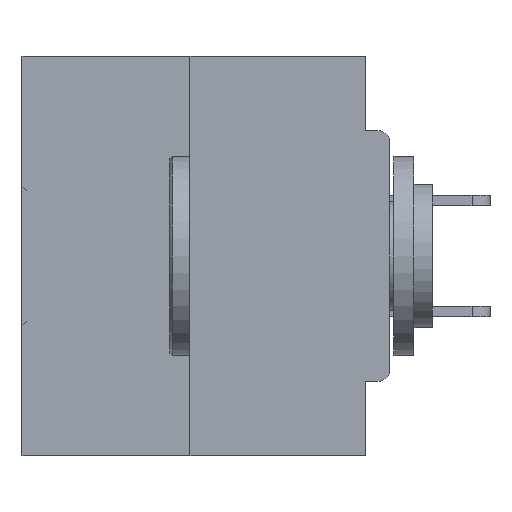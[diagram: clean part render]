
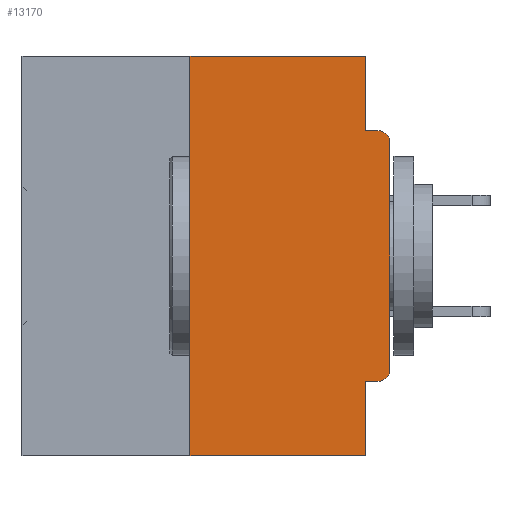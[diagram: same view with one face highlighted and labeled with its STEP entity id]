
A CAD part, left-side view. The second image highlights one B-rep face of the part: STEP entity #13170.
In plain terms, the highlighted planar face has unit normal (-1, 0, 0).
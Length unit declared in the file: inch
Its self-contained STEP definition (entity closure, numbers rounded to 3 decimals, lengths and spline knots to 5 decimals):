
#78 = DIRECTION ( 'NONE',  ( 0., 0., -1. ) ) ;
#475 = EDGE_CURVE ( 'NONE', #14964, #7353, #18288, .T. ) ;
#890 = DIRECTION ( 'NONE',  ( 0., 0., -1. ) ) ;
#1221 = CARTESIAN_POINT ( 'NONE',  ( 0., 0.46, -0.5 ) ) ;
#1668 = EDGE_CURVE ( 'NONE', #23211, #14253, #40710, .T. ) ;
#3344 = EDGE_CURVE ( 'NONE', #44906, #28571, #44698, .T. ) ;
#4486 = AXIS2_PLACEMENT_3D ( 'NONE', #15875, #8685, #5326 ) ;
#4583 = VECTOR ( 'NONE', #78, 39.37008 ) ;
#4726 = LINE ( 'NONE', #22509, #44784 ) ;
#5304 = CARTESIAN_POINT ( 'NONE',  ( 0., 0.25, 0. ) ) ;
#5326 = DIRECTION ( 'NONE',  ( 0., 0., -1. ) ) ;
#5459 = DIRECTION ( 'NONE',  ( 0., 0., 1. ) ) ;
#5738 = CARTESIAN_POINT ( 'NONE',  ( 0., 0.015, -0.1085 ) ) ;
#5760 = LINE ( 'NONE', #10376, #6853 ) ;
#6853 = VECTOR ( 'NONE', #42630, 39.37008 ) ;
#7054 = ORIENTED_EDGE ( 'NONE', *, *, #43190, .F. ) ;
#7353 = VERTEX_POINT ( 'NONE', #10066 ) ;
#8255 = VERTEX_POINT ( 'NONE', #42864 ) ;
#8685 = DIRECTION ( 'NONE',  ( -1., 0., 0. ) ) ;
#8760 = DIRECTION ( 'NONE',  ( 0., -1., 0. ) ) ;
#10066 = CARTESIAN_POINT ( 'NONE',  ( 0., 0.015, -0.0935 ) ) ;
#10376 = CARTESIAN_POINT ( 'NONE',  ( 0., 0.031, 0. ) ) ;
#10467 = VECTOR ( 'NONE', #25319, 39.37008 ) ;
#10963 = ORIENTED_EDGE ( 'NONE', *, *, #11370, .T. ) ;
#11117 = CARTESIAN_POINT ( 'NONE',  ( 0., 0.031, -0.5 ) ) ;
#11202 = DIRECTION ( 'NONE',  ( 0., 1., 0. ) ) ;
#11370 = EDGE_CURVE ( 'NONE', #8255, #14964, #37147, .T. ) ;
#12118 = AXIS2_PLACEMENT_3D ( 'NONE', #5738, #40565, #19067 ) ;
#12357 = EDGE_CURVE ( 'NONE', #30990, #26503, #5760, .T. ) ;
#12519 = LINE ( 'NONE', #40222, #41104 ) ;
#13170 = ADVANCED_FACE ( 'NONE', ( #38039 ), #38951, .F. ) ;
#13207 = ORIENTED_EDGE ( 'NONE', *, *, #20850, .T. ) ;
#14200 = EDGE_CURVE ( 'NONE', #23211, #28475, #35765, .T. ) ;
#14253 = VERTEX_POINT ( 'NONE', #11117 ) ;
#14556 = AXIS2_PLACEMENT_3D ( 'NONE', #17894, #42499, #890 ) ;
#14964 = VERTEX_POINT ( 'NONE', #22464 ) ;
#15875 = CARTESIAN_POINT ( 'NONE',  ( 0., 0.015, -0.3915 ) ) ;
#16377 = CARTESIAN_POINT ( 'NONE',  ( 0., 0.031, 0. ) ) ;
#17894 = CARTESIAN_POINT ( 'NONE',  ( 0., 0.46, 0. ) ) ;
#18135 = ORIENTED_EDGE ( 'NONE', *, *, #3344, .F. ) ;
#18288 = CIRCLE ( 'NONE', #12118, 0.015 ) ;
#19067 = DIRECTION ( 'NONE',  ( 0., 0., -1. ) ) ;
#20060 = CIRCLE ( 'NONE', #4486, 0.015 ) ;
#20195 = ORIENTED_EDGE ( 'NONE', *, *, #475, .T. ) ;
#20850 = EDGE_CURVE ( 'NONE', #44906, #8255, #20060, .T. ) ;
#21730 = ORIENTED_EDGE ( 'NONE', *, *, #38142, .F. ) ;
#22464 = CARTESIAN_POINT ( 'NONE',  ( 0., 0., -0.1085 ) ) ;
#22509 = CARTESIAN_POINT ( 'NONE',  ( 0., 0.46, 0. ) ) ;
#23211 = VERTEX_POINT ( 'NONE', #44111 ) ;
#23949 = CARTESIAN_POINT ( 'NONE',  ( 0., 0.015, -0.4065 ) ) ;
#23973 = VECTOR ( 'NONE', #28690, 39.37008 ) ;
#24333 = LINE ( 'NONE', #42291, #4583 ) ;
#24680 = EDGE_LOOP ( 'NONE', ( #21730, #38659, #35243, #7054, #18135, #13207, #10963, #20195, #37753, #43602 ) ) ;
#25319 = DIRECTION ( 'NONE',  ( 0., -1., 0. ) ) ;
#25388 = EDGE_CURVE ( 'NONE', #26503, #7353, #12519, .T. ) ;
#26503 = VERTEX_POINT ( 'NONE', #33304 ) ;
#28475 = VERTEX_POINT ( 'NONE', #35783 ) ;
#28540 = CARTESIAN_POINT ( 'NONE',  ( 0., 0., 0. ) ) ;
#28571 = VERTEX_POINT ( 'NONE', #31695 ) ;
#28690 = DIRECTION ( 'NONE',  ( 0., 0., 1. ) ) ;
#29555 = DIRECTION ( 'NONE',  ( 0., -1., 0. ) ) ;
#30990 = VERTEX_POINT ( 'NONE', #16377 ) ;
#31695 = CARTESIAN_POINT ( 'NONE',  ( 0., 0.031, -0.4065 ) ) ;
#32264 = CARTESIAN_POINT ( 'NONE',  ( 0., 0., -0.4065 ) ) ;
#33150 = VECTOR ( 'NONE', #11202, 39.37008 ) ;
#33304 = CARTESIAN_POINT ( 'NONE',  ( 0., 0.031, -0.0935 ) ) ;
#35243 = ORIENTED_EDGE ( 'NONE', *, *, #1668, .T. ) ;
#35765 = LINE ( 'NONE', #5304, #43996 ) ;
#35783 = CARTESIAN_POINT ( 'NONE',  ( 0., 0.25, 0. ) ) ;
#37147 = LINE ( 'NONE', #28540, #23973 ) ;
#37753 = ORIENTED_EDGE ( 'NONE', *, *, #25388, .F. ) ;
#38039 = FACE_OUTER_BOUND ( 'NONE', #24680, .T. ) ;
#38142 = EDGE_CURVE ( 'NONE', #28475, #30990, #4726, .T. ) ;
#38659 = ORIENTED_EDGE ( 'NONE', *, *, #14200, .F. ) ;
#38951 = PLANE ( 'NONE',  #14556 ) ;
#40222 = CARTESIAN_POINT ( 'NONE',  ( 0., 0., -0.0935 ) ) ;
#40565 = DIRECTION ( 'NONE',  ( -1., 0., 0. ) ) ;
#40710 = LINE ( 'NONE', #1221, #10467 ) ;
#41104 = VECTOR ( 'NONE', #8760, 39.37008 ) ;
#42291 = CARTESIAN_POINT ( 'NONE',  ( 0., 0.031, -0.5 ) ) ;
#42499 = DIRECTION ( 'NONE',  ( 1., 0., 0. ) ) ;
#42630 = DIRECTION ( 'NONE',  ( 0., 0., -1. ) ) ;
#42864 = CARTESIAN_POINT ( 'NONE',  ( 0., 0., -0.3915 ) ) ;
#43190 = EDGE_CURVE ( 'NONE', #28571, #14253, #24333, .T. ) ;
#43602 = ORIENTED_EDGE ( 'NONE', *, *, #12357, .F. ) ;
#43996 = VECTOR ( 'NONE', #5459, 39.37008 ) ;
#44111 = CARTESIAN_POINT ( 'NONE',  ( 0., 0.25, -0.5 ) ) ;
#44698 = LINE ( 'NONE', #32264, #33150 ) ;
#44784 = VECTOR ( 'NONE', #29555, 39.37008 ) ;
#44906 = VERTEX_POINT ( 'NONE', #23949 ) ;
